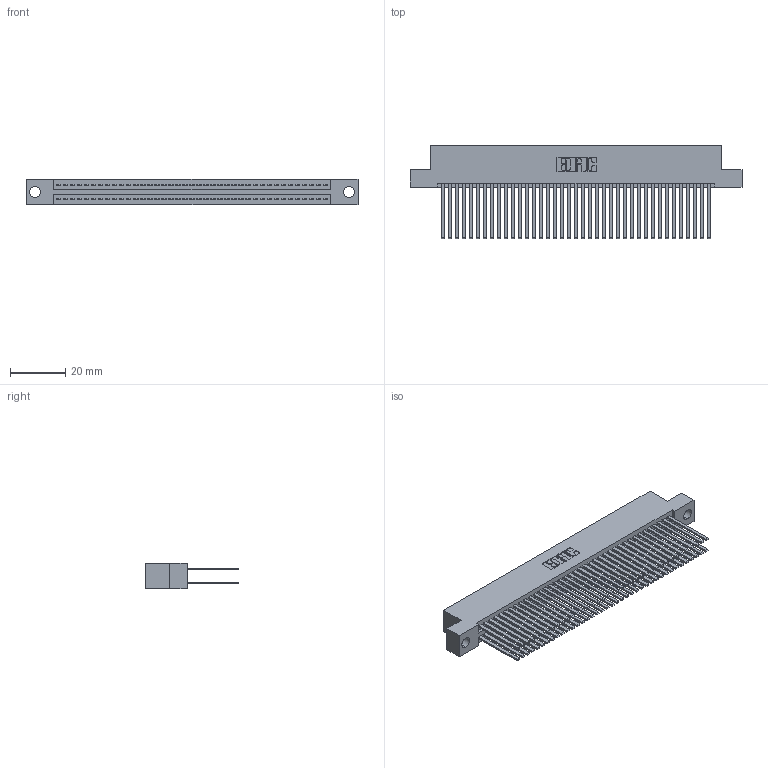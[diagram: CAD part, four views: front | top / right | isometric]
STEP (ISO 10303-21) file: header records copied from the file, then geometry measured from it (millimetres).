
FILE_DESCRIPTION (( 'STEP AP203' ), '1' );
FILE_NAME ('345-078-544-204.STEP', '2021-05-20T10:50:21', ( '' ), ( '' ), 'SwSTEP 2.0', 'SolidWorks 2020', '' );
FILE_SCHEMA (( 'CONFIG_CONTROL_DESIGN' ));
Length unit declared in the file: inch
Products named in the file (3): 345 Part_Flush Mounting Lugs - 0.156 Dia-TI; 345-292-001_345-293-144; 345-078-544-204
Assembly tree (79 placements, depth 2):
  345-078-544-204
    345 Part_Flush Mounting Lugs - 0.156 Dia-TI
    345-292-001_345-293-144  x78
Bounding box: 120.27 x 33.96 x 9.4 mm (x, y, z)
Volume: 12642.7 mm3; surface area: 21686.2 mm2
Topology: 79 solids, 79 shells, 3572 faces, 10595 edges, 6958 vertices
Faces by surface type: plane 2356, cylinder 1216
Entity records: 31239 total; most frequent: CARTESIAN_POINT 5242, ORIENTED_EDGE 5174, DIRECTION 4623, EDGE_CURVE 2587, LINE 2303, VECTOR 2303, VERTEX_POINT 1722, AXIS2_PLACEMENT_3D 1160
